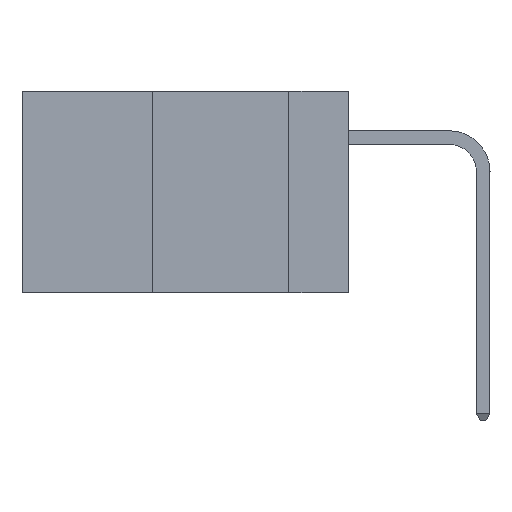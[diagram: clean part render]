
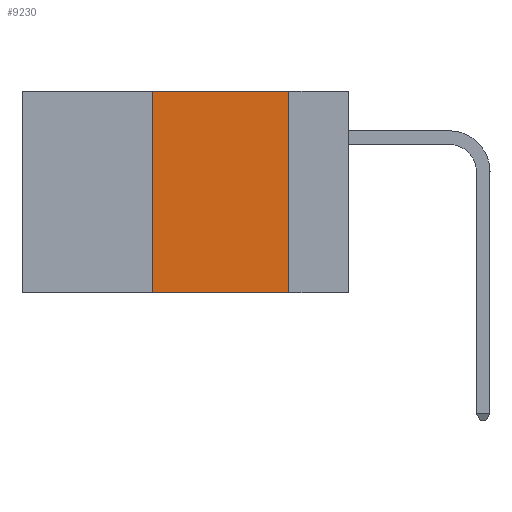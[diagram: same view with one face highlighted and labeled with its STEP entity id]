
A CAD part, left-side view. The second image highlights one B-rep face of the part: STEP entity #9230.
In plain terms, the highlighted planar face has unit normal (-1, 0, 0).
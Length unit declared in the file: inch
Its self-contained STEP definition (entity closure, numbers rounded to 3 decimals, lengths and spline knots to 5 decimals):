
#94 = CARTESIAN_POINT ( 'NONE',  ( 0., 0.36, 0. ) ) ;
#740 = LINE ( 'NONE', #3181, #7679 ) ;
#953 = CARTESIAN_POINT ( 'NONE',  ( 0., 0.11, 0. ) ) ;
#1008 = ORIENTED_EDGE ( 'NONE', *, *, #14360, .F. ) ;
#1136 = CARTESIAN_POINT ( 'NONE',  ( 0., 0.36, 0. ) ) ;
#1165 = CARTESIAN_POINT ( 'NONE',  ( 0., 0.36, -0.37 ) ) ;
#1312 = CARTESIAN_POINT ( 'NONE',  ( 0., 0.11, -0.37 ) ) ;
#1687 = DIRECTION ( 'NONE',  ( 0., -1., 0. ) ) ;
#1761 = CARTESIAN_POINT ( 'NONE',  ( 0., 0.11, 0. ) ) ;
#2323 = VERTEX_POINT ( 'NONE', #94 ) ;
#2631 = DIRECTION ( 'NONE',  ( 0., 0., 1. ) ) ;
#2797 = EDGE_CURVE ( 'NONE', #6602, #2323, #3346, .T. ) ;
#3181 = CARTESIAN_POINT ( 'NONE',  ( 0., 0.6, -0.37 ) ) ;
#3346 = LINE ( 'NONE', #1136, #17085 ) ;
#3756 = EDGE_CURVE ( 'NONE', #12274, #4235, #9540, .T. ) ;
#4235 = VERTEX_POINT ( 'NONE', #1312 ) ;
#5666 = ORIENTED_EDGE ( 'NONE', *, *, #17431, .T. ) ;
#6459 = CARTESIAN_POINT ( 'NONE',  ( 0., 0.6, 0. ) ) ;
#6523 = VECTOR ( 'NONE', #7792, 39.37008 ) ;
#6602 = VERTEX_POINT ( 'NONE', #1165 ) ;
#6699 = DIRECTION ( 'NONE',  ( 0., 0., -1. ) ) ;
#7679 = VECTOR ( 'NONE', #1687, 39.37008 ) ;
#7792 = DIRECTION ( 'NONE',  ( 0., -1., 0. ) ) ;
#8758 = ORIENTED_EDGE ( 'NONE', *, *, #2797, .F. ) ;
#9230 = ADVANCED_FACE ( 'NONE', ( #15486 ), #10576, .F. ) ;
#9540 = LINE ( 'NONE', #1761, #16210 ) ;
#10576 = PLANE ( 'NONE',  #15320 ) ;
#12274 = VERTEX_POINT ( 'NONE', #953 ) ;
#13285 = CARTESIAN_POINT ( 'NONE',  ( 0., 0.6, 0. ) ) ;
#14360 = EDGE_CURVE ( 'NONE', #2323, #12274, #16277, .T. ) ;
#14690 = DIRECTION ( 'NONE',  ( 1., 0., 0. ) ) ;
#15022 = ORIENTED_EDGE ( 'NONE', *, *, #3756, .F. ) ;
#15320 = AXIS2_PLACEMENT_3D ( 'NONE', #13285, #14690, #6699 ) ;
#15486 = FACE_OUTER_BOUND ( 'NONE', #16763, .T. ) ;
#16210 = VECTOR ( 'NONE', #16528, 39.37008 ) ;
#16277 = LINE ( 'NONE', #6459, #6523 ) ;
#16528 = DIRECTION ( 'NONE',  ( 0., 0., -1. ) ) ;
#16763 = EDGE_LOOP ( 'NONE', ( #15022, #1008, #8758, #5666 ) ) ;
#17085 = VECTOR ( 'NONE', #2631, 39.37008 ) ;
#17431 = EDGE_CURVE ( 'NONE', #6602, #4235, #740, .T. ) ;
